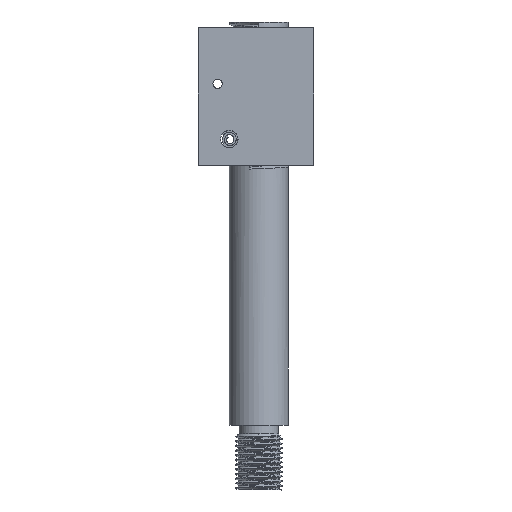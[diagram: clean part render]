
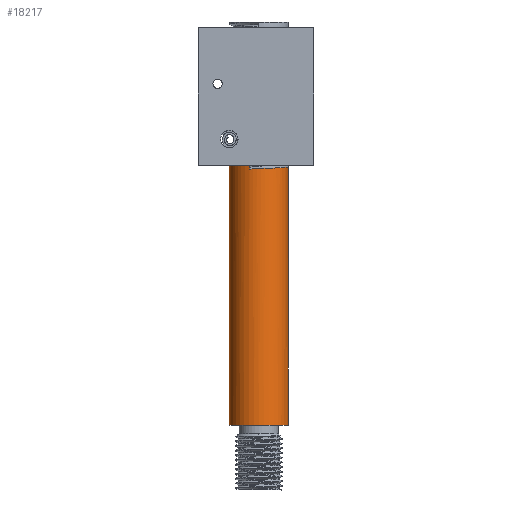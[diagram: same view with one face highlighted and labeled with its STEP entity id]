
A CAD part, left-side view. The second image highlights one B-rep face of the part: STEP entity #18217.
In plain terms, the highlighted cylindrical face has radius 8 mm (diameter 16 mm), a partial arc.
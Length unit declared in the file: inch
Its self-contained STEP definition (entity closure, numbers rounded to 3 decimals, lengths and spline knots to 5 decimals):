
#30 = FACE_OUTER_BOUND ( 'NONE', #21828, .T. ) ;
#237 = ORIENTED_EDGE ( 'NONE', *, *, #28176, .F. ) ;
#732 = CARTESIAN_POINT ( 'NONE',  ( 2.81575, -0.58288, 0.19466 ) ) ;
#870 = EDGE_CURVE ( 'NONE', #11211, #21049, #8643, .T. ) ;
#939 = VERTEX_POINT ( 'NONE', #5813 ) ;
#1768 = CARTESIAN_POINT ( 'NONE',  ( 2.80984, -0.21262, 0.31496 ) ) ;
#1912 = CARTESIAN_POINT ( 'NONE',  ( 2.75079, -0.61451, 0.09733 ) ) ;
#2030 = LINE ( 'NONE', #29230, #27387 ) ;
#2821 = EDGE_CURVE ( 'NONE', #8411, #23260, #21661, .T. ) ;
#3027 = CARTESIAN_POINT ( 'NONE',  ( 2.82362, -0.62992, 0. ) ) ;
#3418 = EDGE_CURVE ( 'NONE', #939, #8411, #2030, .T. ) ;
#3602 = VERTEX_POINT ( 'NONE', #14604 ) ;
#4179 = DIRECTION ( 'NONE',  ( -1., 0., 0. ) ) ;
#4715 = CARTESIAN_POINT ( 'NONE',  ( 2.83346, -0.62992, 0. ) ) ;
#5076 = VERTEX_POINT ( 'NONE', #6590 ) ;
#5638 = CARTESIAN_POINT ( 'NONE',  ( 2.8216, -0.62992, 0.04988 ) ) ;
#5643 = VECTOR ( 'NONE', #29280, 39.37008 ) ;
#5813 = CARTESIAN_POINT ( 'NONE',  ( 2.83346, -0.62992, 0. ) ) ;
#6367 = CARTESIAN_POINT ( 'NONE',  ( 2.82362, -0.62992, 0. ) ) ;
#6381 = DIRECTION ( 'NONE',  ( -1., 0., 0. ) ) ;
#6590 = CARTESIAN_POINT ( 'NONE',  ( 0., 0., 0. ) ) ;
#6847 = CARTESIAN_POINT ( 'NONE',  ( 2.80591, -0.12983, 0.25481 ) ) ;
#7234 = EDGE_CURVE ( 'NONE', #939, #3602, #10883, .T. ) ;
#7579 = CIRCLE ( 'NONE', #32002, 0.31496 ) ;
#7630 = CARTESIAN_POINT ( 'NONE',  ( 2.79409, 0., 0. ) ) ;
#8411 = VERTEX_POINT ( 'NONE', #6367 ) ;
#8643 =( BOUNDED_CURVE ( )  B_SPLINE_CURVE ( 2, ( #24228, #21956, #1912, #11874, #19523, #14647, #29427, #17079, #12825 ),
 .UNSPECIFIED., .F., .T. ) 
 B_SPLINE_CURVE_WITH_KNOTS ( ( 3, 2, 2, 2, 3 ),
 ( 0.9375, 0.94, 0.945, 0.95, 0.9525 ),
 .UNSPECIFIED. ) 
 CURVE ( )  GEOMETRIC_REPRESENTATION_ITEM ( )  RATIONAL_B_SPLINE_CURVE ( ( 0.976, 0.976, 1., 0.951, 1., 0.951, 1., 0.976, 0.976 ) ) 
 REPRESENTATION_ITEM ( '' )  );
#8819 = CARTESIAN_POINT ( 'NONE',  ( 0., -0.31496, 0. ) ) ;
#9292 = ORIENTED_EDGE ( 'NONE', *, *, #7234, .T. ) ;
#9304 = AXIS2_PLACEMENT_3D ( 'NONE', #29985, #22512, #27569 ) ;
#10148 = CYLINDRICAL_SURFACE ( 'NONE', #9304, 0.31496 ) ;
#10378 = CARTESIAN_POINT ( 'NONE',  ( 2.81969, -0.61451, 0.09733 ) ) ;
#10534 = CARTESIAN_POINT ( 'NONE',  ( 2.8, -0.21763, 0.29955 ) ) ;
#10883 =( BOUNDED_CURVE ( )  B_SPLINE_CURVE ( 2, ( #4715, #26545, #14666, #14185, #12212, #22128, #29610, #1768, #6847, #11723, #17260, #27182, #7630 ),
 .UNSPECIFIED., .F., .T. ) 
 B_SPLINE_CURVE_WITH_KNOTS ( ( 3, 2, 2, 2, 2, 2, 3 ),
 ( 0.8875, 0.89, 0.895, 0.9, 0.905, 0.91, 0.9125 ),
 .UNSPECIFIED. ) 
 CURVE ( )  GEOMETRIC_REPRESENTATION_ITEM ( )  RATIONAL_B_SPLINE_CURVE ( ( 0.976, 0.976, 1., 0.951, 1., 0.951, 1., 0.951, 1., 0.951, 1., 0.976, 0.976 ) ) 
 REPRESENTATION_ITEM ( '' )  );
#11211 = VERTEX_POINT ( 'NONE', #31981 ) ;
#11723 = CARTESIAN_POINT ( 'NONE',  ( 2.80197, -0.04704, 0.19466 ) ) ;
#11859 = VERTEX_POINT ( 'NONE', #25374 ) ;
#11860 = DIRECTION ( 'NONE',  ( -1., 0., 0. ) ) ;
#11874 = CARTESIAN_POINT ( 'NONE',  ( 2.74685, -0.58288, 0.19466 ) ) ;
#12212 = CARTESIAN_POINT ( 'NONE',  ( 2.82165, -0.50009, 0.25481 ) ) ;
#12825 = CARTESIAN_POINT ( 'NONE',  ( 2.7311, -0.21763, 0.29955 ) ) ;
#13475 = ORIENTED_EDGE ( 'NONE', *, *, #870, .T. ) ;
#14185 = CARTESIAN_POINT ( 'NONE',  ( 2.82559, -0.58288, 0.19466 ) ) ;
#14604 = CARTESIAN_POINT ( 'NONE',  ( 2.79409, 0., 0. ) ) ;
#14647 = CARTESIAN_POINT ( 'NONE',  ( 2.73898, -0.4173, 0.31496 ) ) ;
#14666 = CARTESIAN_POINT ( 'NONE',  ( 2.82953, -0.61451, 0.09733 ) ) ;
#15242 = LINE ( 'NONE', #22869, #5643 ) ;
#15431 = CARTESIAN_POINT ( 'NONE',  ( 2.80394, -0.31496, 0.31496 ) ) ;
#15747 = CARTESIAN_POINT ( 'NONE',  ( 2.81181, -0.50009, 0.25481 ) ) ;
#16010 = VECTOR ( 'NONE', #4179, 39.37008 ) ;
#16196 = ORIENTED_EDGE ( 'NONE', *, *, #3418, .F. ) ;
#17079 = CARTESIAN_POINT ( 'NONE',  ( 2.73312, -0.26508, 0.31496 ) ) ;
#17260 = CARTESIAN_POINT ( 'NONE',  ( 2.79803, -0.01542, 0.09733 ) ) ;
#17306 = ORIENTED_EDGE ( 'NONE', *, *, #26303, .T. ) ;
#17447 = EDGE_CURVE ( 'NONE', #21049, #23260, #15242, .T. ) ;
#18217 = ADVANCED_FACE ( 'NONE', ( #30 ), #10148, .T. ) ;
#18520 = CARTESIAN_POINT ( 'NONE',  ( 4.3, 0., 0. ) ) ;
#19042 = CARTESIAN_POINT ( 'NONE',  ( 2.8, -0.21763, 0.29955 ) ) ;
#19352 = LINE ( 'NONE', #21780, #24336 ) ;
#19523 = CARTESIAN_POINT ( 'NONE',  ( 2.74291, -0.50009, 0.25481 ) ) ;
#19870 = DIRECTION ( 'NONE',  ( 0., -1., 0. ) ) ;
#21049 = VERTEX_POINT ( 'NONE', #28121 ) ;
#21211 = ORIENTED_EDGE ( 'NONE', *, *, #2821, .F. ) ;
#21661 =( BOUNDED_CURVE ( )  B_SPLINE_CURVE ( 2, ( #3027, #5638, #10378, #732, #15747, #27633, #15431, #28116, #10534 ),
 .UNSPECIFIED., .F., .T. ) 
 B_SPLINE_CURVE_WITH_KNOTS ( ( 3, 2, 2, 2, 3 ),
 ( 0.9375, 0.94, 0.945, 0.95, 0.9525 ),
 .UNSPECIFIED. ) 
 CURVE ( )  GEOMETRIC_REPRESENTATION_ITEM ( )  RATIONAL_B_SPLINE_CURVE ( ( 0.976, 0.976, 1., 0.951, 1., 0.951, 1., 0.976, 0.976 ) ) 
 REPRESENTATION_ITEM ( '' )  );
#21780 = CARTESIAN_POINT ( 'NONE',  ( 4.3, -0.62992, 0. ) ) ;
#21828 = EDGE_LOOP ( 'NONE', ( #9292, #17306, #26681, #237, #13475, #26763, #21211, #16196 ) ) ;
#21956 = CARTESIAN_POINT ( 'NONE',  ( 2.75271, -0.62992, 0.04988 ) ) ;
#22128 = CARTESIAN_POINT ( 'NONE',  ( 2.81772, -0.4173, 0.31496 ) ) ;
#22512 = DIRECTION ( 'NONE',  ( -1., 0., 0. ) ) ;
#22869 = CARTESIAN_POINT ( 'NONE',  ( 4.3, -0.21763, 0.29955 ) ) ;
#23260 = VERTEX_POINT ( 'NONE', #19042 ) ;
#23710 = LINE ( 'NONE', #18520, #16010 ) ;
#24228 = CARTESIAN_POINT ( 'NONE',  ( 2.75472, -0.62992, 0. ) ) ;
#24336 = VECTOR ( 'NONE', #11860, 39.37008 ) ;
#24389 = EDGE_CURVE ( 'NONE', #11859, #5076, #7579, .T. ) ;
#25374 = CARTESIAN_POINT ( 'NONE',  ( 0., -0.62992, 0. ) ) ;
#26303 = EDGE_CURVE ( 'NONE', #3602, #5076, #23710, .T. ) ;
#26545 = CARTESIAN_POINT ( 'NONE',  ( 2.83145, -0.62992, 0.04988 ) ) ;
#26681 = ORIENTED_EDGE ( 'NONE', *, *, #24389, .F. ) ;
#26763 = ORIENTED_EDGE ( 'NONE', *, *, #17447, .T. ) ;
#27182 = CARTESIAN_POINT ( 'NONE',  ( 2.79611, 0., 0.04988 ) ) ;
#27387 = VECTOR ( 'NONE', #29381, 39.37008 ) ;
#27569 = DIRECTION ( 'NONE',  ( 0., -1., 0. ) ) ;
#27633 = CARTESIAN_POINT ( 'NONE',  ( 2.80787, -0.4173, 0.31496 ) ) ;
#28116 = CARTESIAN_POINT ( 'NONE',  ( 2.80202, -0.26508, 0.31496 ) ) ;
#28121 = CARTESIAN_POINT ( 'NONE',  ( 2.7311, -0.21763, 0.29955 ) ) ;
#28176 = EDGE_CURVE ( 'NONE', #11211, #11859, #19352, .T. ) ;
#29230 = CARTESIAN_POINT ( 'NONE',  ( 4.3, -0.62992, 0. ) ) ;
#29280 = DIRECTION ( 'NONE',  ( 1., 0., 0. ) ) ;
#29381 = DIRECTION ( 'NONE',  ( -1., 0., 0. ) ) ;
#29427 = CARTESIAN_POINT ( 'NONE',  ( 2.73504, -0.31496, 0.31496 ) ) ;
#29610 = CARTESIAN_POINT ( 'NONE',  ( 2.81378, -0.31496, 0.31496 ) ) ;
#29985 = CARTESIAN_POINT ( 'NONE',  ( 4.3, -0.31496, 0. ) ) ;
#31981 = CARTESIAN_POINT ( 'NONE',  ( 2.75472, -0.62992, 0. ) ) ;
#32002 = AXIS2_PLACEMENT_3D ( 'NONE', #8819, #6381, #19870 ) ;
